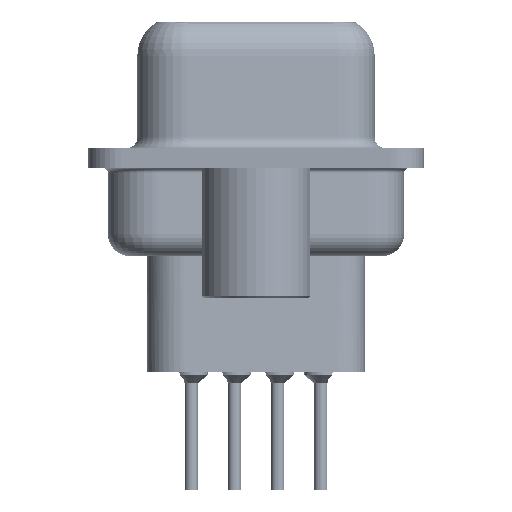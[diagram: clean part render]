
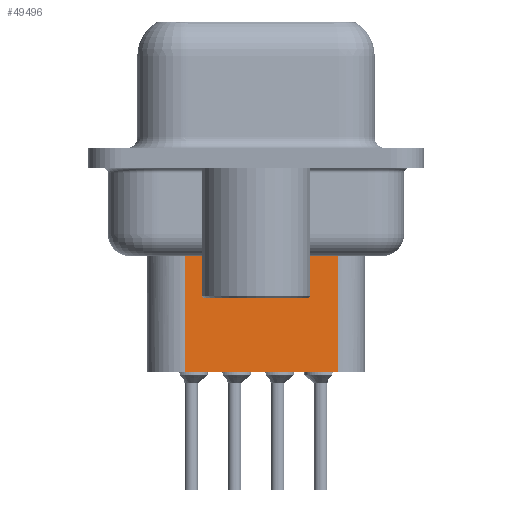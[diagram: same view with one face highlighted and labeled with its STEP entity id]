
A CAD part, left-side view. The second image highlights one B-rep face of the part: STEP entity #49496.
In plain terms, the highlighted planar face has unit normal (-0.985, -0.174, 0).
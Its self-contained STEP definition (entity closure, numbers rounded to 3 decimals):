
#796 = CARTESIAN_POINT ( 'NONE',  ( 4.624, 3.24, -3.1 ) ) ;
#1292 = CARTESIAN_POINT ( 'NONE',  ( 4.624, 3.24, -3.975 ) ) ;
#4609 = DIRECTION ( 'NONE',  ( 0.174, -0.985, 0. ) ) ;
#4903 = CARTESIAN_POINT ( 'NONE',  ( 5.858, -3.76, -3.975 ) ) ;
#4931 = VECTOR ( 'NONE', #34585, 1000. ) ;
#6124 = CARTESIAN_POINT ( 'NONE',  ( 4.624, 3.24, -3.1 ) ) ;
#7256 = EDGE_CURVE ( 'NONE', #36752, #26501, #37386, .T. ) ;
#9711 = CARTESIAN_POINT ( 'NONE',  ( 5.858, -3.76, -3.1 ) ) ;
#13554 = LINE ( 'NONE', #9711, #17141 ) ;
#13656 = ORIENTED_EDGE ( 'NONE', *, *, #34853, .F. ) ;
#17141 = VECTOR ( 'NONE', #40093, 1000. ) ;
#17401 = VECTOR ( 'NONE', #47145, 1000. ) ;
#18550 = LINE ( 'NONE', #36539, #18584 ) ;
#18584 = VECTOR ( 'NONE', #19915, 1000. ) ;
#19056 = PLANE ( 'NONE',  #38996 ) ;
#19684 = EDGE_CURVE ( 'NONE', #25120, #57128, #13554, .T. ) ;
#19915 = DIRECTION ( 'NONE',  ( -0.174, 0.985, 0. ) ) ;
#20046 = ORIENTED_EDGE ( 'NONE', *, *, #19684, .F. ) ;
#22334 = EDGE_LOOP ( 'NONE', ( #20046, #27904, #27922, #13656 ) ) ;
#25120 = VERTEX_POINT ( 'NONE', #4903 ) ;
#26501 = VERTEX_POINT ( 'NONE', #39573 ) ;
#26871 = CARTESIAN_POINT ( 'NONE',  ( 4.453, 4.209, -3.975 ) ) ;
#27904 = ORIENTED_EDGE ( 'NONE', *, *, #40947, .T. ) ;
#27922 = ORIENTED_EDGE ( 'NONE', *, *, #7256, .T. ) ;
#34585 = DIRECTION ( 'NONE',  ( -0.174, 0.985, 0. ) ) ;
#34853 = EDGE_CURVE ( 'NONE', #57128, #26501, #18550, .T. ) ;
#36447 = DIRECTION ( 'NONE',  ( -0.985, -0.174, 0. ) ) ;
#36539 = CARTESIAN_POINT ( 'NONE',  ( 4.624, 3.24, -9.85 ) ) ;
#36752 = VERTEX_POINT ( 'NONE', #1292 ) ;
#37386 = LINE ( 'NONE', #6124, #17401 ) ;
#38996 = AXIS2_PLACEMENT_3D ( 'NONE', #796, #36447, #4609 ) ;
#39573 = CARTESIAN_POINT ( 'NONE',  ( 4.624, 3.24, -9.85 ) ) ;
#40060 = CARTESIAN_POINT ( 'NONE',  ( 5.858, -3.76, -9.85 ) ) ;
#40093 = DIRECTION ( 'NONE',  ( 0., 0., -1. ) ) ;
#40947 = EDGE_CURVE ( 'NONE', #25120, #36752, #48759, .T. ) ;
#47145 = DIRECTION ( 'NONE',  ( 0., 0., -1. ) ) ;
#48759 = LINE ( 'NONE', #26871, #4931 ) ;
#49496 = ADVANCED_FACE ( 'NONE', ( #55024 ), #19056, .T. ) ;
#55024 = FACE_OUTER_BOUND ( 'NONE', #22334, .T. ) ;
#57128 = VERTEX_POINT ( 'NONE', #40060 ) ;
